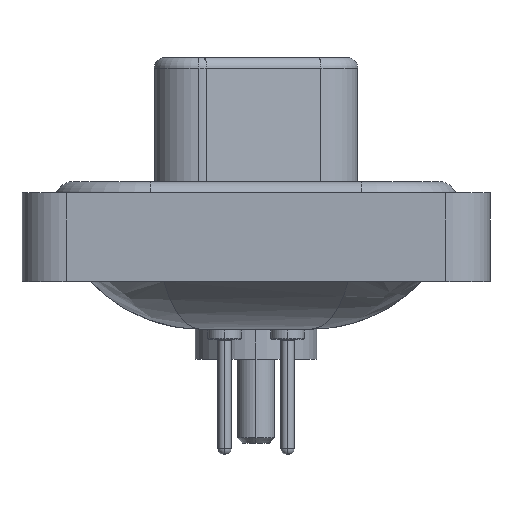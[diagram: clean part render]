
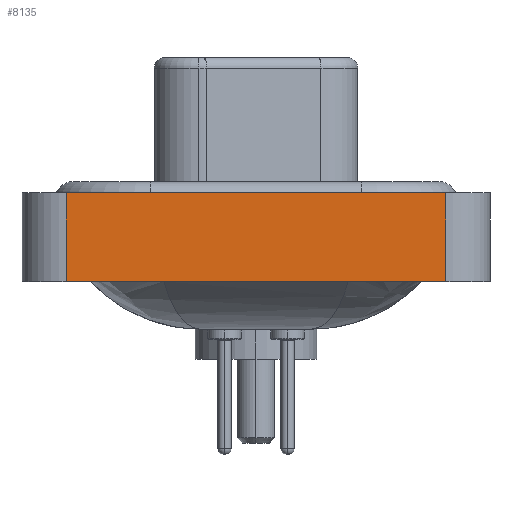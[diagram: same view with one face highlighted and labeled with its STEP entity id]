
A CAD part, left-side view. The second image highlights one B-rep face of the part: STEP entity #8135.
In plain terms, the highlighted planar face has unit normal (-1, 0, 0).
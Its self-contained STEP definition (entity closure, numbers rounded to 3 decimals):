
#637 = CARTESIAN_POINT ( 'NONE',  ( -7.35, 8.55, -3.6 ) ) ;
#1526 = EDGE_LOOP ( 'NONE', ( #10638, #20738, #16608, #3677 ) ) ;
#1720 = CARTESIAN_POINT ( 'NONE',  ( -7.35, -8.55, -3.6 ) ) ;
#2612 = AXIS2_PLACEMENT_3D ( 'NONE', #1720, #23774, #12913 ) ;
#3633 = VERTEX_POINT ( 'NONE', #6677 ) ;
#3677 = ORIENTED_EDGE ( 'NONE', *, *, #10657, .T. ) ;
#4383 = VECTOR ( 'NONE', #14616, 1000. ) ;
#5221 = VECTOR ( 'NONE', #17820, 1000. ) ;
#5284 = VERTEX_POINT ( 'NONE', #637 ) ;
#6324 = DIRECTION ( 'NONE',  ( 0., -1., 0. ) ) ;
#6677 = CARTESIAN_POINT ( 'NONE',  ( -7.35, -8.55, 0.4 ) ) ;
#7044 = DIRECTION ( 'NONE',  ( 0., 0., 1. ) ) ;
#7107 = VERTEX_POINT ( 'NONE', #10642 ) ;
#7113 = VERTEX_POINT ( 'NONE', #17004 ) ;
#8135 = ADVANCED_FACE ( 'NONE', ( #9363 ), #16836, .T. ) ;
#8873 = LINE ( 'NONE', #23768, #19264 ) ;
#9363 = FACE_OUTER_BOUND ( 'NONE', #1526, .T. ) ;
#9890 = EDGE_CURVE ( 'NONE', #7107, #3633, #15815, .T. ) ;
#10638 = ORIENTED_EDGE ( 'NONE', *, *, #20616, .T. ) ;
#10642 = CARTESIAN_POINT ( 'NONE',  ( -7.35, 8.55, 0.4 ) ) ;
#10657 = EDGE_CURVE ( 'NONE', #5284, #7113, #11303, .T. ) ;
#11303 = LINE ( 'NONE', #20220, #4383 ) ;
#12031 = CARTESIAN_POINT ( 'NONE',  ( -7.35, -8.55, 0.4 ) ) ;
#12913 = DIRECTION ( 'NONE',  ( 0., 0., 1. ) ) ;
#14616 = DIRECTION ( 'NONE',  ( 0., -1., 0. ) ) ;
#15815 = LINE ( 'NONE', #12031, #23420 ) ;
#15878 = LINE ( 'NONE', #17363, #5221 ) ;
#16608 = ORIENTED_EDGE ( 'NONE', *, *, #18415, .F. ) ;
#16836 = PLANE ( 'NONE',  #2612 ) ;
#17004 = CARTESIAN_POINT ( 'NONE',  ( -7.35, -8.55, -3.6 ) ) ;
#17363 = CARTESIAN_POINT ( 'NONE',  ( -7.35, -8.55, -3.6 ) ) ;
#17820 = DIRECTION ( 'NONE',  ( 0., 0., 1. ) ) ;
#18415 = EDGE_CURVE ( 'NONE', #5284, #7107, #8873, .T. ) ;
#19264 = VECTOR ( 'NONE', #7044, 1000. ) ;
#20220 = CARTESIAN_POINT ( 'NONE',  ( -7.35, -8.55, -3.6 ) ) ;
#20616 = EDGE_CURVE ( 'NONE', #7113, #3633, #15878, .T. ) ;
#20738 = ORIENTED_EDGE ( 'NONE', *, *, #9890, .F. ) ;
#23420 = VECTOR ( 'NONE', #6324, 1000. ) ;
#23768 = CARTESIAN_POINT ( 'NONE',  ( -7.35, 8.55, -3.6 ) ) ;
#23774 = DIRECTION ( 'NONE',  ( -1., 0., 0. ) ) ;
